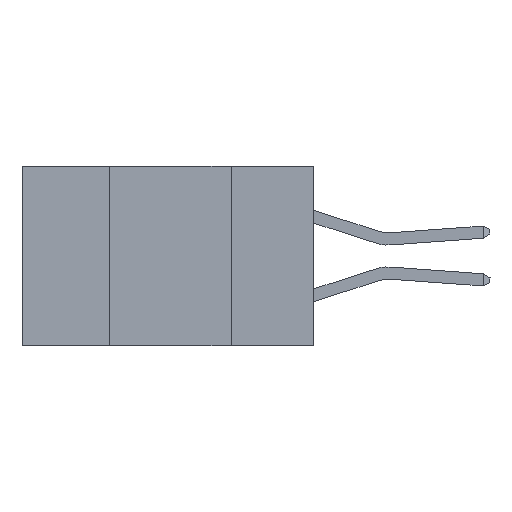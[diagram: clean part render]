
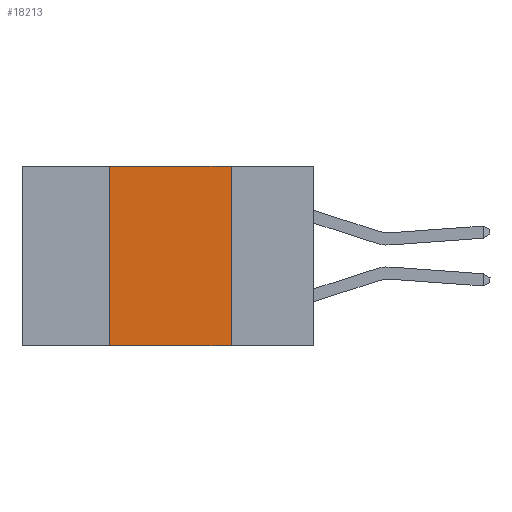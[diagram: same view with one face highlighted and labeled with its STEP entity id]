
A CAD part, left-side view. The second image highlights one B-rep face of the part: STEP entity #18213.
In plain terms, the highlighted planar face has unit normal (-1, 0, 0).
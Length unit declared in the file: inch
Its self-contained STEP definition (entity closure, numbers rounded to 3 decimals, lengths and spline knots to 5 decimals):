
#1348 = CARTESIAN_POINT ( 'NONE',  ( 0., 0.42, 0. ) ) ;
#3140 = DIRECTION ( 'NONE',  ( 1., 0., 0. ) ) ;
#6674 = VERTEX_POINT ( 'NONE', #41528 ) ;
#7510 = CARTESIAN_POINT ( 'NONE',  ( 0., 0.6, 0. ) ) ;
#8638 = LINE ( 'NONE', #42196, #17697 ) ;
#9992 = VERTEX_POINT ( 'NONE', #18607 ) ;
#12246 = LINE ( 'NONE', #15430, #33643 ) ;
#12873 = AXIS2_PLACEMENT_3D ( 'NONE', #40635, #3140, #27017 ) ;
#14840 = DIRECTION ( 'NONE',  ( 0., -1., 0. ) ) ;
#15313 = VECTOR ( 'NONE', #25376, 39.37008 ) ;
#15430 = CARTESIAN_POINT ( 'NONE',  ( 0., 0.17, 0. ) ) ;
#16560 = EDGE_CURVE ( 'NONE', #9992, #38133, #20545, .T. ) ;
#17697 = VECTOR ( 'NONE', #14840, 39.37008 ) ;
#18213 = ADVANCED_FACE ( 'NONE', ( #24667 ), #44066, .F. ) ;
#18245 = VERTEX_POINT ( 'NONE', #20298 ) ;
#18607 = CARTESIAN_POINT ( 'NONE',  ( 0., 0.42, 0. ) ) ;
#19627 = EDGE_LOOP ( 'NONE', ( #23543, #26704, #39086, #27292 ) ) ;
#20298 = CARTESIAN_POINT ( 'NONE',  ( 0., 0.17, -0.37 ) ) ;
#20545 = LINE ( 'NONE', #7510, #37678 ) ;
#23543 = ORIENTED_EDGE ( 'NONE', *, *, #27085, .F. ) ;
#24411 = LINE ( 'NONE', #1348, #15313 ) ;
#24667 = FACE_OUTER_BOUND ( 'NONE', #19627, .T. ) ;
#25060 = EDGE_CURVE ( 'NONE', #6674, #18245, #8638, .T. ) ;
#25376 = DIRECTION ( 'NONE',  ( 0., 0., 1. ) ) ;
#26704 = ORIENTED_EDGE ( 'NONE', *, *, #16560, .F. ) ;
#27017 = DIRECTION ( 'NONE',  ( 0., 0., -1. ) ) ;
#27085 = EDGE_CURVE ( 'NONE', #38133, #18245, #12246, .T. ) ;
#27292 = ORIENTED_EDGE ( 'NONE', *, *, #25060, .T. ) ;
#28768 = EDGE_CURVE ( 'NONE', #6674, #9992, #24411, .T. ) ;
#31330 = DIRECTION ( 'NONE',  ( 0., -1., 0. ) ) ;
#33049 = CARTESIAN_POINT ( 'NONE',  ( 0., 0.17, 0. ) ) ;
#33643 = VECTOR ( 'NONE', #39398, 39.37008 ) ;
#37678 = VECTOR ( 'NONE', #31330, 39.37008 ) ;
#38133 = VERTEX_POINT ( 'NONE', #33049 ) ;
#39086 = ORIENTED_EDGE ( 'NONE', *, *, #28768, .F. ) ;
#39398 = DIRECTION ( 'NONE',  ( 0., 0., -1. ) ) ;
#40635 = CARTESIAN_POINT ( 'NONE',  ( 0., 0.6, 0. ) ) ;
#41528 = CARTESIAN_POINT ( 'NONE',  ( 0., 0.42, -0.37 ) ) ;
#42196 = CARTESIAN_POINT ( 'NONE',  ( 0., 0.6, -0.37 ) ) ;
#44066 = PLANE ( 'NONE',  #12873 ) ;
